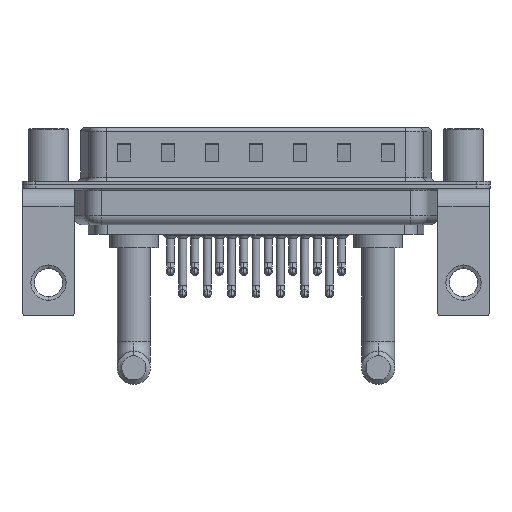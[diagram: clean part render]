
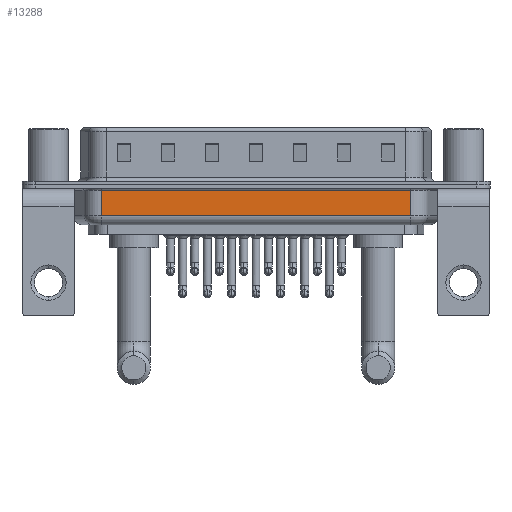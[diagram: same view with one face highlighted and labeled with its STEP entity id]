
A CAD part, front view. The second image highlights one B-rep face of the part: STEP entity #13288.
In plain terms, the highlighted planar face has unit normal (0, -1, 0).
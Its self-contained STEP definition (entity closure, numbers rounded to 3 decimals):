
#262 = CARTESIAN_POINT ( 'NONE',  ( 6.006, -5.35, -4.5 ) ) ;
#1161 = VERTEX_POINT ( 'NONE', #10025 ) ;
#1431 = ORIENTED_EDGE ( 'NONE', *, *, #20203, .T. ) ;
#2260 = CARTESIAN_POINT ( 'NONE',  ( 6.006, -5.35, -0.65 ) ) ;
#2502 = VECTOR ( 'NONE', #25239, 1000. ) ;
#2559 = ORIENTED_EDGE ( 'NONE', *, *, #23938, .F. ) ;
#2739 = DIRECTION ( 'NONE',  ( 0., 0., 1. ) ) ;
#3318 = EDGE_LOOP ( 'NONE', ( #2559, #1431, #8523, #11604 ) ) ;
#3420 = DIRECTION ( 'NONE',  ( 0., 0., 1. ) ) ;
#5080 = CARTESIAN_POINT ( 'NONE',  ( 41.044, -5.35, -4.5 ) ) ;
#5231 = VERTEX_POINT ( 'NONE', #24465 ) ;
#6145 = CARTESIAN_POINT ( 'NONE',  ( 6.006, -5.35, -3.5 ) ) ;
#8337 = LINE ( 'NONE', #6145, #11520 ) ;
#8523 = ORIENTED_EDGE ( 'NONE', *, *, #26851, .T. ) ;
#8683 = CARTESIAN_POINT ( 'NONE',  ( 6.006, -5.35, -4.5 ) ) ;
#9399 = VERTEX_POINT ( 'NONE', #14655 ) ;
#10025 = CARTESIAN_POINT ( 'NONE',  ( 41.044, -5.35, -3.5 ) ) ;
#10040 = AXIS2_PLACEMENT_3D ( 'NONE', #262, #23698, #2739 ) ;
#10660 = DIRECTION ( 'NONE',  ( -1., 0., 0. ) ) ;
#11520 = VECTOR ( 'NONE', #12859, 1000. ) ;
#11604 = ORIENTED_EDGE ( 'NONE', *, *, #20207, .T. ) ;
#12364 = VERTEX_POINT ( 'NONE', #26970 ) ;
#12859 = DIRECTION ( 'NONE',  ( 1., 0., 0. ) ) ;
#13288 = ADVANCED_FACE ( 'NONE', ( #21620 ), #19416, .F. ) ;
#14655 = CARTESIAN_POINT ( 'NONE',  ( 6.006, -5.35, -0.65 ) ) ;
#14940 = VECTOR ( 'NONE', #3420, 1000. ) ;
#16601 = LINE ( 'NONE', #2260, #17244 ) ;
#17244 = VECTOR ( 'NONE', #10660, 1000. ) ;
#19416 = PLANE ( 'NONE',  #10040 ) ;
#20203 = EDGE_CURVE ( 'NONE', #12364, #1161, #8337, .T. ) ;
#20207 = EDGE_CURVE ( 'NONE', #5231, #9399, #16601, .T. ) ;
#20828 = LINE ( 'NONE', #8683, #2502 ) ;
#21620 = FACE_OUTER_BOUND ( 'NONE', #3318, .T. ) ;
#23698 = DIRECTION ( 'NONE',  ( 0., 1., 0. ) ) ;
#23938 = EDGE_CURVE ( 'NONE', #12364, #9399, #20828, .T. ) ;
#23962 = LINE ( 'NONE', #5080, #14940 ) ;
#24465 = CARTESIAN_POINT ( 'NONE',  ( 41.044, -5.35, -0.65 ) ) ;
#25239 = DIRECTION ( 'NONE',  ( 0., 0., 1. ) ) ;
#26851 = EDGE_CURVE ( 'NONE', #1161, #5231, #23962, .T. ) ;
#26970 = CARTESIAN_POINT ( 'NONE',  ( 6.006, -5.35, -3.5 ) ) ;
